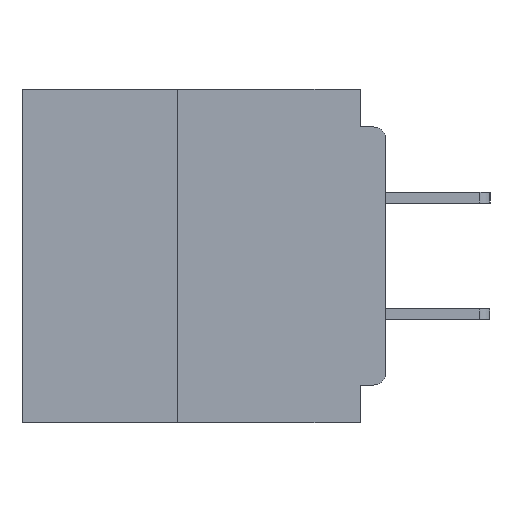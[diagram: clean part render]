
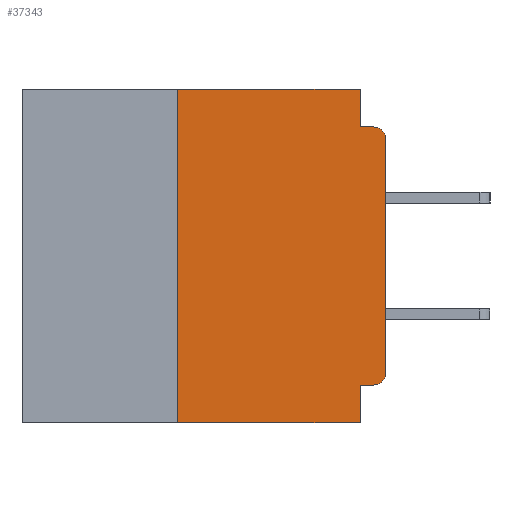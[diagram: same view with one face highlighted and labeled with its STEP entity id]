
A CAD part, left-side view. The second image highlights one B-rep face of the part: STEP entity #37343.
In plain terms, the highlighted planar face has unit normal (-1, 0, 0).
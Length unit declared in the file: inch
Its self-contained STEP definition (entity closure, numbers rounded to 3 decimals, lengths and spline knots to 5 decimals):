
#12 = CARTESIAN_POINT ( 'NONE',  ( 0., 0.031, 0. ) ) ;
#173 = VERTEX_POINT ( 'NONE', #11363 ) ;
#1227 = ORIENTED_EDGE ( 'NONE', *, *, #21547, .F. ) ;
#1256 = VECTOR ( 'NONE', #40287, 39.37008 ) ;
#2963 = FACE_OUTER_BOUND ( 'NONE', #26255, .T. ) ;
#3049 = VECTOR ( 'NONE', #9961, 39.37008 ) ;
#4363 = ORIENTED_EDGE ( 'NONE', *, *, #4417, .F. ) ;
#4417 = EDGE_CURVE ( 'NONE', #44164, #12483, #12601, .T. ) ;
#6191 = CARTESIAN_POINT ( 'NONE',  ( 0., 0.25, -0.4 ) ) ;
#6221 = DIRECTION ( 'NONE',  ( -1., 0., 0. ) ) ;
#7103 = EDGE_CURVE ( 'NONE', #173, #43747, #36989, .T. ) ;
#7871 = EDGE_CURVE ( 'NONE', #29686, #30826, #52217, .T. ) ;
#8343 = PLANE ( 'NONE',  #28300 ) ;
#9536 = CARTESIAN_POINT ( 'NONE',  ( 0., 0., -0.355 ) ) ;
#9961 = DIRECTION ( 'NONE',  ( 0., -1., 0. ) ) ;
#11363 = CARTESIAN_POINT ( 'NONE',  ( 0., 0.015, -0.355 ) ) ;
#11830 = VERTEX_POINT ( 'NONE', #47818 ) ;
#12483 = VERTEX_POINT ( 'NONE', #39368 ) ;
#12601 = LINE ( 'NONE', #6191, #1256 ) ;
#13459 = ORIENTED_EDGE ( 'NONE', *, *, #7103, .T. ) ;
#13521 = VECTOR ( 'NONE', #27662, 39.37008 ) ;
#14043 = CARTESIAN_POINT ( 'NONE',  ( 0., 0.437, -0.4 ) ) ;
#14047 = EDGE_CURVE ( 'NONE', #19110, #11830, #27318, .T. ) ;
#14375 = LINE ( 'NONE', #14043, #3049 ) ;
#14607 = EDGE_CURVE ( 'NONE', #173, #19110, #32675, .T. ) ;
#16621 = CARTESIAN_POINT ( 'NONE',  ( 0., 0., -0.34 ) ) ;
#16861 = CARTESIAN_POINT ( 'NONE',  ( 0., 0.437, 0. ) ) ;
#16863 = EDGE_CURVE ( 'NONE', #44164, #11830, #14375, .T. ) ;
#18169 = VECTOR ( 'NONE', #44282, 39.37008 ) ;
#19110 = VERTEX_POINT ( 'NONE', #37858 ) ;
#19948 = VECTOR ( 'NONE', #22811, 39.37008 ) ;
#20923 = VERTEX_POINT ( 'NONE', #12 ) ;
#21035 = CARTESIAN_POINT ( 'NONE',  ( 0., 0.031, 0. ) ) ;
#21050 = EDGE_CURVE ( 'NONE', #43747, #49979, #55177, .T. ) ;
#21164 = DIRECTION ( 'NONE',  ( 0., 0., -1. ) ) ;
#21547 = EDGE_CURVE ( 'NONE', #20923, #29686, #43825, .T. ) ;
#21790 = CARTESIAN_POINT ( 'NONE',  ( 0., 0.015, -0.34 ) ) ;
#22811 = DIRECTION ( 'NONE',  ( 0., 0., -1. ) ) ;
#23392 = CARTESIAN_POINT ( 'NONE',  ( 0., 0.437, 0. ) ) ;
#25699 = ORIENTED_EDGE ( 'NONE', *, *, #50070, .F. ) ;
#26093 = DIRECTION ( 'NONE',  ( 0., 0., -1. ) ) ;
#26255 = EDGE_LOOP ( 'NONE', ( #50792, #27113, #38077, #1227, #25699, #4363, #30286, #26602, #45593, #13459 ) ) ;
#26602 = ORIENTED_EDGE ( 'NONE', *, *, #14047, .F. ) ;
#26821 = CARTESIAN_POINT ( 'NONE',  ( 0., 0.015, -0.045 ) ) ;
#27113 = ORIENTED_EDGE ( 'NONE', *, *, #35695, .T. ) ;
#27318 = LINE ( 'NONE', #44049, #19948 ) ;
#27662 = DIRECTION ( 'NONE',  ( 0., -1., 0. ) ) ;
#27796 = CARTESIAN_POINT ( 'NONE',  ( 0., 0.25, -0.4 ) ) ;
#28300 = AXIS2_PLACEMENT_3D ( 'NONE', #16861, #46730, #21164 ) ;
#29686 = VERTEX_POINT ( 'NONE', #52791 ) ;
#30286 = ORIENTED_EDGE ( 'NONE', *, *, #16863, .T. ) ;
#30826 = VERTEX_POINT ( 'NONE', #26821 ) ;
#31763 = CARTESIAN_POINT ( 'NONE',  ( 0., 0.015, -0.06 ) ) ;
#31818 = AXIS2_PLACEMENT_3D ( 'NONE', #31763, #6221, #36061 ) ;
#31861 = CIRCLE ( 'NONE', #31818, 0.015 ) ;
#32675 = LINE ( 'NONE', #9536, #42666 ) ;
#33703 = AXIS2_PLACEMENT_3D ( 'NONE', #21790, #51611, #26093 ) ;
#35235 = DIRECTION ( 'NONE',  ( 0., 1., 0. ) ) ;
#35514 = CARTESIAN_POINT ( 'NONE',  ( 0., 0., -0.06 ) ) ;
#35695 = EDGE_CURVE ( 'NONE', #49979, #30826, #31861, .T. ) ;
#36061 = DIRECTION ( 'NONE',  ( 0., 0., -1. ) ) ;
#36989 = CIRCLE ( 'NONE', #33703, 0.015 ) ;
#37343 = ADVANCED_FACE ( 'NONE', ( #2963 ), #8343, .F. ) ;
#37858 = CARTESIAN_POINT ( 'NONE',  ( 0., 0.031, -0.355 ) ) ;
#38077 = ORIENTED_EDGE ( 'NONE', *, *, #7871, .F. ) ;
#38397 = DIRECTION ( 'NONE',  ( 0., 0., -1. ) ) ;
#39188 = CARTESIAN_POINT ( 'NONE',  ( 0., 0., 0. ) ) ;
#39368 = CARTESIAN_POINT ( 'NONE',  ( 0., 0.25, 0. ) ) ;
#40287 = DIRECTION ( 'NONE',  ( 0., 0., 1. ) ) ;
#42480 = VECTOR ( 'NONE', #38397, 39.37008 ) ;
#42666 = VECTOR ( 'NONE', #35235, 39.37008 ) ;
#43747 = VERTEX_POINT ( 'NONE', #16621 ) ;
#43825 = LINE ( 'NONE', #21035, #42480 ) ;
#43885 = VECTOR ( 'NONE', #52036, 39.37008 ) ;
#44049 = CARTESIAN_POINT ( 'NONE',  ( 0., 0.031, -0.4 ) ) ;
#44164 = VERTEX_POINT ( 'NONE', #27796 ) ;
#44282 = DIRECTION ( 'NONE',  ( 0., -1., 0. ) ) ;
#45593 = ORIENTED_EDGE ( 'NONE', *, *, #14607, .F. ) ;
#46730 = DIRECTION ( 'NONE',  ( 1., 0., 0. ) ) ;
#47556 = LINE ( 'NONE', #23392, #13521 ) ;
#47818 = CARTESIAN_POINT ( 'NONE',  ( 0., 0.031, -0.4 ) ) ;
#48575 = CARTESIAN_POINT ( 'NONE',  ( 0., 0., -0.045 ) ) ;
#49979 = VERTEX_POINT ( 'NONE', #35514 ) ;
#50070 = EDGE_CURVE ( 'NONE', #12483, #20923, #47556, .T. ) ;
#50792 = ORIENTED_EDGE ( 'NONE', *, *, #21050, .T. ) ;
#51611 = DIRECTION ( 'NONE',  ( -1., 0., 0. ) ) ;
#52036 = DIRECTION ( 'NONE',  ( 0., 0., 1. ) ) ;
#52217 = LINE ( 'NONE', #48575, #18169 ) ;
#52791 = CARTESIAN_POINT ( 'NONE',  ( 0., 0.031, -0.045 ) ) ;
#55177 = LINE ( 'NONE', #39188, #43885 ) ;
